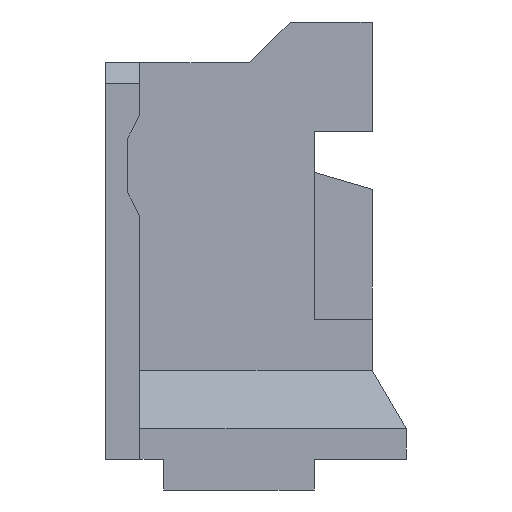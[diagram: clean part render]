
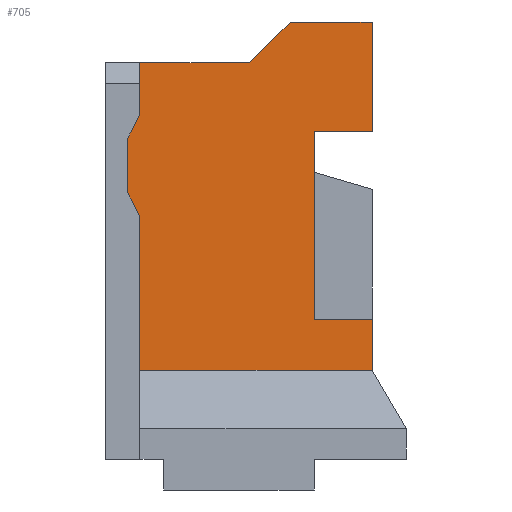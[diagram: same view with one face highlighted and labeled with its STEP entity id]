
A CAD part, left-side view. The second image highlights one B-rep face of the part: STEP entity #705.
In plain terms, the highlighted planar face has unit normal (-1, 0, 0).
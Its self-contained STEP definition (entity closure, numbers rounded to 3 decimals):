
#57 = LINE ( 'NONE', #7725, #1663 ) ;
#74 = VECTOR ( 'NONE', #5256, 1000. ) ;
#97 = VECTOR ( 'NONE', #1300, 1000. ) ;
#116 = CARTESIAN_POINT ( 'NONE',  ( -1.25, 1.1, -4.5 ) ) ;
#187 = EDGE_CURVE ( 'NONE', #10534, #9745, #8033, .T. ) ;
#289 = CARTESIAN_POINT ( 'NONE',  ( -1.25, -2.3, -4.5 ) ) ;
#322 = DIRECTION ( 'NONE',  ( 0., -1., 0. ) ) ;
#431 = ORIENTED_EDGE ( 'NONE', *, *, #8015, .F. ) ;
#549 = ORIENTED_EDGE ( 'NONE', *, *, #9242, .F. ) ;
#705 = ADVANCED_FACE ( 'NONE', ( #4629 ), #6837, .F. ) ;
#723 = VECTOR ( 'NONE', #925, 1000. ) ;
#869 = LINE ( 'NONE', #4017, #9703 ) ;
#925 = DIRECTION ( 'NONE',  ( 0., 1., 0. ) ) ;
#1102 = CARTESIAN_POINT ( 'NONE',  ( -1.25, 1.1, -0.75 ) ) ;
#1300 = DIRECTION ( 'NONE',  ( 0., 0., 1. ) ) ;
#1357 = CARTESIAN_POINT ( 'NONE',  ( -1.25, 1.275, -1.9 ) ) ;
#1392 = VERTEX_POINT ( 'NONE', #5942 ) ;
#1410 = CARTESIAN_POINT ( 'NONE',  ( -1.25, -1.45, -1. ) ) ;
#1473 = CARTESIAN_POINT ( 'NONE',  ( -1.25, -1.45, -1. ) ) ;
#1517 = LINE ( 'NONE', #8213, #8486 ) ;
#1639 = VERTEX_POINT ( 'NONE', #2920 ) ;
#1663 = VECTOR ( 'NONE', #8531, 1000. ) ;
#1684 = EDGE_CURVE ( 'NONE', #8259, #1392, #5936, .T. ) ;
#1858 = VERTEX_POINT ( 'NONE', #1410 ) ;
#1892 = ORIENTED_EDGE ( 'NONE', *, *, #3934, .F. ) ;
#2258 = EDGE_CURVE ( 'NONE', #9744, #8763, #4504, .T. ) ;
#2325 = EDGE_CURVE ( 'NONE', #1639, #10534, #3526, .T. ) ;
#2663 = CARTESIAN_POINT ( 'NONE',  ( -1.25, -3., -4.5 ) ) ;
#2667 = ORIENTED_EDGE ( 'NONE', *, *, #6017, .F. ) ;
#2785 = EDGE_CURVE ( 'NONE', #6007, #10473, #869, .T. ) ;
#2920 = CARTESIAN_POINT ( 'NONE',  ( -1.25, -1.45, -3.75 ) ) ;
#3094 = VECTOR ( 'NONE', #8788, 1000. ) ;
#3125 = CARTESIAN_POINT ( 'NONE',  ( -1.25, 1.1, 0. ) ) ;
#3187 = VERTEX_POINT ( 'NONE', #9746 ) ;
#3307 = EDGE_CURVE ( 'NONE', #1858, #1639, #5240, .T. ) ;
#3387 = ORIENTED_EDGE ( 'NONE', *, *, #2325, .F. ) ;
#3526 = LINE ( 'NONE', #6308, #8790 ) ;
#3689 = ORIENTED_EDGE ( 'NONE', *, *, #9023, .F. ) ;
#3820 = ORIENTED_EDGE ( 'NONE', *, *, #7054, .F. ) ;
#3908 = DIRECTION ( 'NONE',  ( 0., 0., -1. ) ) ;
#3923 = LINE ( 'NONE', #3125, #5273 ) ;
#3934 = EDGE_CURVE ( 'NONE', #3187, #1858, #4553, .T. ) ;
#4017 = CARTESIAN_POINT ( 'NONE',  ( -1.25, 1.1, -0.75 ) ) ;
#4052 = DIRECTION ( 'NONE',  ( 0., -1., 0. ) ) ;
#4152 = DIRECTION ( 'NONE',  ( 1., 0., 0. ) ) ;
#4197 = VERTEX_POINT ( 'NONE', #1357 ) ;
#4252 = ORIENTED_EDGE ( 'NONE', *, *, #2258, .F. ) ;
#4504 = LINE ( 'NONE', #10416, #4880 ) ;
#4549 = ORIENTED_EDGE ( 'NONE', *, *, #2785, .F. ) ;
#4553 = LINE ( 'NONE', #7400, #5346 ) ;
#4629 = FACE_OUTER_BOUND ( 'NONE', #9133, .T. ) ;
#4880 = VECTOR ( 'NONE', #322, 1000. ) ;
#5042 = DIRECTION ( 'NONE',  ( 0., 0.447, 0.894 ) ) ;
#5240 = LINE ( 'NONE', #1473, #5498 ) ;
#5242 = LINE ( 'NONE', #2663, #723 ) ;
#5256 = DIRECTION ( 'NONE',  ( 0., 0., -1. ) ) ;
#5273 = VECTOR ( 'NONE', #4052, 1000. ) ;
#5346 = VECTOR ( 'NONE', #9860, 1000. ) ;
#5498 = VECTOR ( 'NONE', #3908, 1000. ) ;
#5619 = LINE ( 'NONE', #10511, #3094 ) ;
#5936 = LINE ( 'NONE', #6318, #97 ) ;
#5942 = CARTESIAN_POINT ( 'NONE',  ( -1.25, 1.1, -2.25 ) ) ;
#6007 = VERTEX_POINT ( 'NONE', #7318 ) ;
#6017 = EDGE_CURVE ( 'NONE', #10473, #6188, #8127, .T. ) ;
#6159 = CARTESIAN_POINT ( 'NONE',  ( -1.25, -2.3, 0.6 ) ) ;
#6188 = VERTEX_POINT ( 'NONE', #10846 ) ;
#6308 = CARTESIAN_POINT ( 'NONE',  ( -1.25, 3.057, -3.75 ) ) ;
#6318 = CARTESIAN_POINT ( 'NONE',  ( -1.25, 1.1, -5.8 ) ) ;
#6672 = CARTESIAN_POINT ( 'NONE',  ( -1.25, -2.3, -3.75 ) ) ;
#6733 = CARTESIAN_POINT ( 'NONE',  ( -1.25, 0., 0. ) ) ;
#6837 = PLANE ( 'NONE',  #8891 ) ;
#7005 = CARTESIAN_POINT ( 'NONE',  ( -1.25, -2.3, -1.85 ) ) ;
#7054 = EDGE_CURVE ( 'NONE', #4197, #6007, #57, .T. ) ;
#7275 = ORIENTED_EDGE ( 'NONE', *, *, #187, .F. ) ;
#7318 = CARTESIAN_POINT ( 'NONE',  ( -1.25, 1.275, -1.1 ) ) ;
#7387 = VECTOR ( 'NONE', #7954, 1000. ) ;
#7400 = CARTESIAN_POINT ( 'NONE',  ( -1.25, -2.3, -1. ) ) ;
#7658 = ORIENTED_EDGE ( 'NONE', *, *, #1684, .F. ) ;
#7725 = CARTESIAN_POINT ( 'NONE',  ( -1.25, 1.275, -2.25 ) ) ;
#7826 = ORIENTED_EDGE ( 'NONE', *, *, #8195, .F. ) ;
#7850 = ORIENTED_EDGE ( 'NONE', *, *, #3307, .F. ) ;
#7954 = DIRECTION ( 'NONE',  ( 0., 0., -1. ) ) ;
#8015 = EDGE_CURVE ( 'NONE', #6188, #8965, #3923, .T. ) ;
#8033 = LINE ( 'NONE', #7005, #7387 ) ;
#8127 = LINE ( 'NONE', #10658, #10634 ) ;
#8195 = EDGE_CURVE ( 'NONE', #8763, #3187, #9325, .T. ) ;
#8213 = CARTESIAN_POINT ( 'NONE',  ( -1.25, 1.1, -2.25 ) ) ;
#8259 = VERTEX_POINT ( 'NONE', #116 ) ;
#8441 = DIRECTION ( 'NONE',  ( 0., 0., -1. ) ) ;
#8460 = DIRECTION ( 'NONE',  ( 0., -0.447, 0.894 ) ) ;
#8486 = VECTOR ( 'NONE', #5042, 1000. ) ;
#8531 = DIRECTION ( 'NONE',  ( 0., 0., 1. ) ) ;
#8666 = CARTESIAN_POINT ( 'NONE',  ( -1.25, -2.3, 0.6 ) ) ;
#8763 = VERTEX_POINT ( 'NONE', #8666 ) ;
#8788 = DIRECTION ( 'NONE',  ( 0., -0.707, 0.707 ) ) ;
#8790 = VECTOR ( 'NONE', #8800, 1000. ) ;
#8800 = DIRECTION ( 'NONE',  ( 0., -1., 0. ) ) ;
#8891 = AXIS2_PLACEMENT_3D ( 'NONE', #6733, #4152, #8441 ) ;
#8965 = VERTEX_POINT ( 'NONE', #10131 ) ;
#9023 = EDGE_CURVE ( 'NONE', #9745, #8259, #5242, .T. ) ;
#9039 = DIRECTION ( 'NONE',  ( 0., 0., 1. ) ) ;
#9133 = EDGE_LOOP ( 'NONE', ( #2667, #4549, #3820, #9798, #7658, #3689, #7275, #3387, #7850, #1892, #7826, #4252, #549, #431 ) ) ;
#9242 = EDGE_CURVE ( 'NONE', #8965, #9744, #5619, .T. ) ;
#9259 = CARTESIAN_POINT ( 'NONE',  ( -1.25, -1.1, 0.6 ) ) ;
#9325 = LINE ( 'NONE', #6159, #74 ) ;
#9453 = EDGE_CURVE ( 'NONE', #1392, #4197, #1517, .T. ) ;
#9703 = VECTOR ( 'NONE', #8460, 1000. ) ;
#9744 = VERTEX_POINT ( 'NONE', #9259 ) ;
#9745 = VERTEX_POINT ( 'NONE', #289 ) ;
#9746 = CARTESIAN_POINT ( 'NONE',  ( -1.25, -2.3, -1. ) ) ;
#9798 = ORIENTED_EDGE ( 'NONE', *, *, #9453, .F. ) ;
#9860 = DIRECTION ( 'NONE',  ( 0., 1., 0. ) ) ;
#10131 = CARTESIAN_POINT ( 'NONE',  ( -1.25, -0.5, 0. ) ) ;
#10416 = CARTESIAN_POINT ( 'NONE',  ( -1.25, -1.1, 0.6 ) ) ;
#10473 = VERTEX_POINT ( 'NONE', #1102 ) ;
#10511 = CARTESIAN_POINT ( 'NONE',  ( -1.25, -0.5, 0. ) ) ;
#10534 = VERTEX_POINT ( 'NONE', #6672 ) ;
#10634 = VECTOR ( 'NONE', #9039, 1000. ) ;
#10658 = CARTESIAN_POINT ( 'NONE',  ( -1.25, 1.1, -5.8 ) ) ;
#10846 = CARTESIAN_POINT ( 'NONE',  ( -1.25, 1.1, 0. ) ) ;
